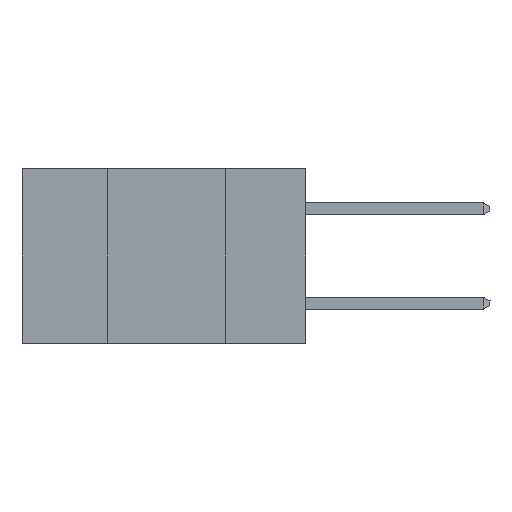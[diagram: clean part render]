
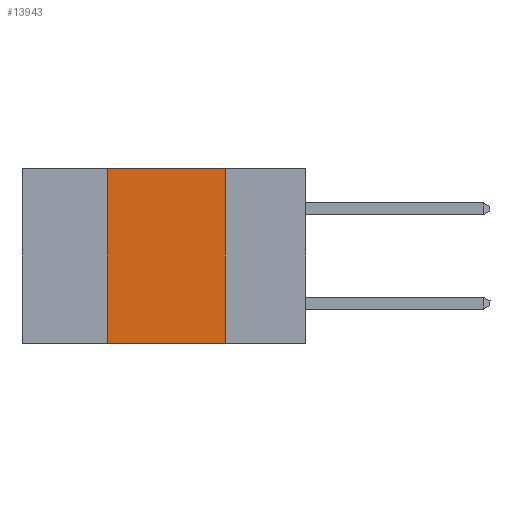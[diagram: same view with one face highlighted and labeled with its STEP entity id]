
A CAD part, left-side view. The second image highlights one B-rep face of the part: STEP entity #13943.
In plain terms, the highlighted planar face has unit normal (-1, 0, 0).
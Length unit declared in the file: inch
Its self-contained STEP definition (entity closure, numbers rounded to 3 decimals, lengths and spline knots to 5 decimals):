
#5 = LINE ( 'NONE', #12036, #10530 ) ;
#41 = CARTESIAN_POINT ( 'NONE',  ( 0., 0.42, 0. ) ) ;
#238 = CARTESIAN_POINT ( 'NONE',  ( 0., 0.6, -0.37 ) ) ;
#2108 = CARTESIAN_POINT ( 'NONE',  ( 0., 0.42, 0. ) ) ;
#2688 = EDGE_CURVE ( 'NONE', #12866, #6234, #3192, .T. ) ;
#2703 = VECTOR ( 'NONE', #12939, 39.37008 ) ;
#3032 = DIRECTION ( 'NONE',  ( 0., 0., -1. ) ) ;
#3192 = LINE ( 'NONE', #238, #10806 ) ;
#3388 = CARTESIAN_POINT ( 'NONE',  ( 0., 0.17, -0.37 ) ) ;
#3398 = VERTEX_POINT ( 'NONE', #2108 ) ;
#3984 = ORIENTED_EDGE ( 'NONE', *, *, #4649, .F. ) ;
#4012 = DIRECTION ( 'NONE',  ( 0., 0., -1. ) ) ;
#4140 = ORIENTED_EDGE ( 'NONE', *, *, #10144, .F. ) ;
#4309 = PLANE ( 'NONE',  #13199 ) ;
#4649 = EDGE_CURVE ( 'NONE', #12866, #3398, #5042, .T. ) ;
#5042 = LINE ( 'NONE', #41, #15133 ) ;
#5728 = VERTEX_POINT ( 'NONE', #8156 ) ;
#6234 = VERTEX_POINT ( 'NONE', #3388 ) ;
#6900 = FACE_OUTER_BOUND ( 'NONE', #12673, .T. ) ;
#8111 = DIRECTION ( 'NONE',  ( 0., -1., 0. ) ) ;
#8113 = ORIENTED_EDGE ( 'NONE', *, *, #13923, .F. ) ;
#8156 = CARTESIAN_POINT ( 'NONE',  ( 0., 0.17, 0. ) ) ;
#10144 = EDGE_CURVE ( 'NONE', #3398, #5728, #11351, .T. ) ;
#10491 = CARTESIAN_POINT ( 'NONE',  ( 0., 0.6, 0. ) ) ;
#10530 = VECTOR ( 'NONE', #4012, 39.37008 ) ;
#10806 = VECTOR ( 'NONE', #8111, 39.37008 ) ;
#11351 = LINE ( 'NONE', #10491, #2703 ) ;
#12036 = CARTESIAN_POINT ( 'NONE',  ( 0., 0.17, 0. ) ) ;
#12673 = EDGE_LOOP ( 'NONE', ( #8113, #4140, #3984, #13227 ) ) ;
#12866 = VERTEX_POINT ( 'NONE', #16147 ) ;
#12939 = DIRECTION ( 'NONE',  ( 0., -1., 0. ) ) ;
#13199 = AXIS2_PLACEMENT_3D ( 'NONE', #16066, #16189, #3032 ) ;
#13227 = ORIENTED_EDGE ( 'NONE', *, *, #2688, .T. ) ;
#13923 = EDGE_CURVE ( 'NONE', #5728, #6234, #5, .T. ) ;
#13943 = ADVANCED_FACE ( 'NONE', ( #6900 ), #4309, .F. ) ;
#15133 = VECTOR ( 'NONE', #16050, 39.37008 ) ;
#16050 = DIRECTION ( 'NONE',  ( 0., 0., 1. ) ) ;
#16066 = CARTESIAN_POINT ( 'NONE',  ( 0., 0.6, 0. ) ) ;
#16147 = CARTESIAN_POINT ( 'NONE',  ( 0., 0.42, -0.37 ) ) ;
#16189 = DIRECTION ( 'NONE',  ( 1., 0., 0. ) ) ;
